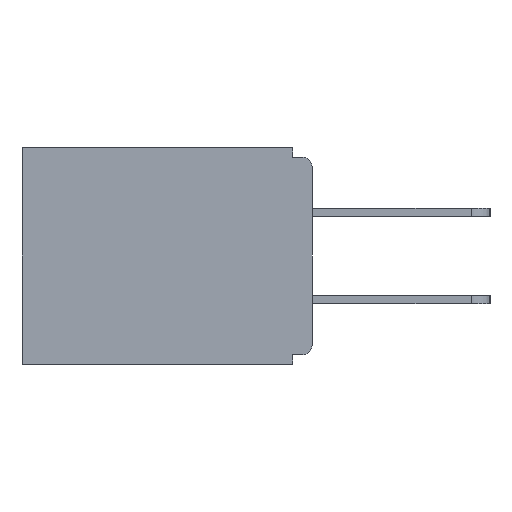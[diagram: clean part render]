
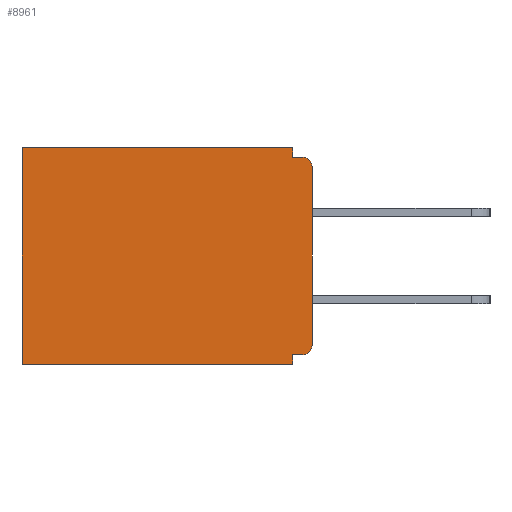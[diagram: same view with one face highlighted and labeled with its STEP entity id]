
A CAD part, left-side view. The second image highlights one B-rep face of the part: STEP entity #8961.
In plain terms, the highlighted planar face has unit normal (-1, 0, 0).
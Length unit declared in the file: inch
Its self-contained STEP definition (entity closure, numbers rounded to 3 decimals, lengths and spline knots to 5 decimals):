
#93 = VERTEX_POINT ( 'NONE', #8154 ) ;
#167 = VERTEX_POINT ( 'NONE', #8464 ) ;
#208 = CARTESIAN_POINT ( 'NONE',  ( 0.298, 0., -0.03 ) ) ;
#242 = EDGE_CURVE ( 'NONE', #7669, #3308, #11118, .T. ) ;
#282 = LINE ( 'NONE', #7850, #13154 ) ;
#484 = CARTESIAN_POINT ( 'NONE',  ( 0.298, 0.031, -0.343 ) ) ;
#503 = LINE ( 'NONE', #8533, #9941 ) ;
#682 = VECTOR ( 'NONE', #1915, 39.37008 ) ;
#713 = ORIENTED_EDGE ( 'NONE', *, *, #13412, .T. ) ;
#1222 = ORIENTED_EDGE ( 'NONE', *, *, #10885, .F. ) ;
#1343 = CARTESIAN_POINT ( 'NONE',  ( 0.298, 0., 0. ) ) ;
#1388 = CARTESIAN_POINT ( 'NONE',  ( 0.298, 0., 0. ) ) ;
#1451 = CARTESIAN_POINT ( 'NONE',  ( 0.298, 0.46, -0.343 ) ) ;
#1731 = VECTOR ( 'NONE', #11656, 39.37008 ) ;
#1915 = DIRECTION ( 'NONE',  ( 0., 1., 0. ) ) ;
#1954 = VECTOR ( 'NONE', #4701, 39.37008 ) ;
#2103 = VERTEX_POINT ( 'NONE', #208 ) ;
#2361 = LINE ( 'NONE', #1388, #13104 ) ;
#2614 = ORIENTED_EDGE ( 'NONE', *, *, #12274, .T. ) ;
#2644 = CARTESIAN_POINT ( 'NONE',  ( 0.298, 0.015, -0.313 ) ) ;
#2751 = CARTESIAN_POINT ( 'NONE',  ( 0.298, 0.031, -0.343 ) ) ;
#2826 = CARTESIAN_POINT ( 'NONE',  ( 0.298, 0.031, -0.015 ) ) ;
#3034 = FACE_OUTER_BOUND ( 'NONE', #10890, .T. ) ;
#3101 = AXIS2_PLACEMENT_3D ( 'NONE', #5116, #13346, #4937 ) ;
#3112 = EDGE_CURVE ( 'NONE', #10198, #6564, #7614, .T. ) ;
#3141 = CARTESIAN_POINT ( 'NONE',  ( 0.298, 0.031, 0. ) ) ;
#3308 = VERTEX_POINT ( 'NONE', #2826 ) ;
#3719 = ORIENTED_EDGE ( 'NONE', *, *, #7777, .F. ) ;
#3832 = LINE ( 'NONE', #2751, #7221 ) ;
#4027 = CARTESIAN_POINT ( 'NONE',  ( 0.298, 0.031, -0.328 ) ) ;
#4072 = ORIENTED_EDGE ( 'NONE', *, *, #3112, .F. ) ;
#4126 = AXIS2_PLACEMENT_3D ( 'NONE', #2644, #8791, #6720 ) ;
#4187 = ORIENTED_EDGE ( 'NONE', *, *, #9193, .T. ) ;
#4283 = EDGE_CURVE ( 'NONE', #2103, #93, #2361, .T. ) ;
#4674 = DIRECTION ( 'NONE',  ( 0., 0., -1. ) ) ;
#4701 = DIRECTION ( 'NONE',  ( 0., 1., 0. ) ) ;
#4905 = VERTEX_POINT ( 'NONE', #4027 ) ;
#4937 = DIRECTION ( 'NONE',  ( 0., 0., -1. ) ) ;
#5116 = CARTESIAN_POINT ( 'NONE',  ( 0.298, 0.015, -0.03 ) ) ;
#5133 = VERTEX_POINT ( 'NONE', #7450 ) ;
#5185 = ORIENTED_EDGE ( 'NONE', *, *, #12097, .F. ) ;
#5441 = CARTESIAN_POINT ( 'NONE',  ( 0.298, 0., -0.343 ) ) ;
#5442 = DIRECTION ( 'NONE',  ( 0., 0., -1. ) ) ;
#5500 = VERTEX_POINT ( 'NONE', #12110 ) ;
#6206 = CIRCLE ( 'NONE', #3101, 0.015 ) ;
#6244 = LINE ( 'NONE', #13302, #682 ) ;
#6564 = VERTEX_POINT ( 'NONE', #1451 ) ;
#6720 = DIRECTION ( 'NONE',  ( 0., 0., -1. ) ) ;
#6787 = CARTESIAN_POINT ( 'NONE',  ( 0.298, 0., 0. ) ) ;
#7221 = VECTOR ( 'NONE', #7429, 39.37008 ) ;
#7429 = DIRECTION ( 'NONE',  ( 0., 0., -1. ) ) ;
#7450 = CARTESIAN_POINT ( 'NONE',  ( 0.298, 0.015, -0.015 ) ) ;
#7592 = DIRECTION ( 'NONE',  ( 0., 0., -1. ) ) ;
#7614 = LINE ( 'NONE', #5441, #1731 ) ;
#7669 = VERTEX_POINT ( 'NONE', #3141 ) ;
#7777 = EDGE_CURVE ( 'NONE', #3308, #5133, #282, .T. ) ;
#7850 = CARTESIAN_POINT ( 'NONE',  ( 0.298, 0., -0.015 ) ) ;
#8154 = CARTESIAN_POINT ( 'NONE',  ( 0.298, 0., -0.313 ) ) ;
#8464 = CARTESIAN_POINT ( 'NONE',  ( 0.298, 0.015, -0.328 ) ) ;
#8533 = CARTESIAN_POINT ( 'NONE',  ( 0.298, 0.46, 0. ) ) ;
#8601 = PLANE ( 'NONE',  #9584 ) ;
#8791 = DIRECTION ( 'NONE',  ( -1., 0., 0. ) ) ;
#8961 = ADVANCED_FACE ( 'NONE', ( #3034 ), #8601, .F. ) ;
#9190 = ORIENTED_EDGE ( 'NONE', *, *, #12358, .T. ) ;
#9193 = EDGE_CURVE ( 'NONE', #167, #93, #10000, .T. ) ;
#9501 = DIRECTION ( 'NONE',  ( 1., 0., 0. ) ) ;
#9584 = AXIS2_PLACEMENT_3D ( 'NONE', #1343, #9501, #4674 ) ;
#9671 = VECTOR ( 'NONE', #12885, 39.37008 ) ;
#9941 = VECTOR ( 'NONE', #5442, 39.37008 ) ;
#10000 = CIRCLE ( 'NONE', #4126, 0.015 ) ;
#10198 = VERTEX_POINT ( 'NONE', #12303 ) ;
#10509 = ORIENTED_EDGE ( 'NONE', *, *, #4283, .F. ) ;
#10885 = EDGE_CURVE ( 'NONE', #4905, #10198, #3832, .T. ) ;
#10890 = EDGE_LOOP ( 'NONE', ( #713, #3719, #13017, #9190, #2614, #4072, #1222, #5185, #4187, #10509 ) ) ;
#11118 = LINE ( 'NONE', #484, #9671 ) ;
#11656 = DIRECTION ( 'NONE',  ( 0., 1., 0. ) ) ;
#11734 = LINE ( 'NONE', #6787, #1954 ) ;
#12068 = DIRECTION ( 'NONE',  ( 0., -1., 0. ) ) ;
#12097 = EDGE_CURVE ( 'NONE', #167, #4905, #6244, .T. ) ;
#12110 = CARTESIAN_POINT ( 'NONE',  ( 0.298, 0.46, 0. ) ) ;
#12274 = EDGE_CURVE ( 'NONE', #5500, #6564, #503, .T. ) ;
#12303 = CARTESIAN_POINT ( 'NONE',  ( 0.298, 0.031, -0.343 ) ) ;
#12358 = EDGE_CURVE ( 'NONE', #7669, #5500, #11734, .T. ) ;
#12885 = DIRECTION ( 'NONE',  ( 0., 0., -1. ) ) ;
#13017 = ORIENTED_EDGE ( 'NONE', *, *, #242, .F. ) ;
#13104 = VECTOR ( 'NONE', #7592, 39.37008 ) ;
#13154 = VECTOR ( 'NONE', #12068, 39.37008 ) ;
#13302 = CARTESIAN_POINT ( 'NONE',  ( 0.298, 0., -0.328 ) ) ;
#13346 = DIRECTION ( 'NONE',  ( -1., 0., 0. ) ) ;
#13412 = EDGE_CURVE ( 'NONE', #2103, #5133, #6206, .T. ) ;
